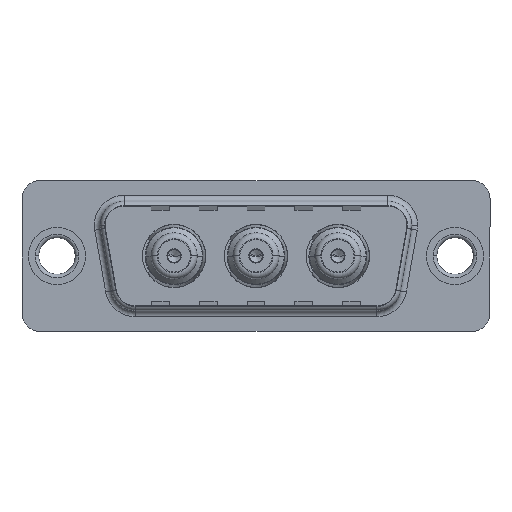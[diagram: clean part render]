
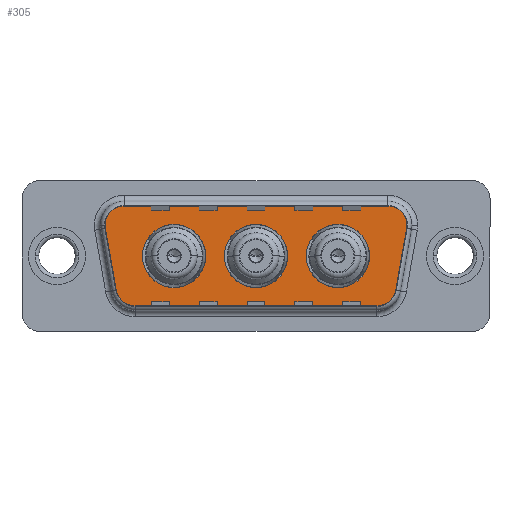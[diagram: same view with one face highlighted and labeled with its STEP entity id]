
A CAD part, top view. The second image highlights one B-rep face of the part: STEP entity #305.
In plain terms, the highlighted planar face has unit normal (0, 0, 1).
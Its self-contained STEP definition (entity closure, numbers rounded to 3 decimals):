
#219 = CIRCLE ( 'NONE', #7672, 2. ) ;
#305 = ADVANCED_FACE ( 'NONE', ( #7602, #4813, #5475, #1991 ), #2094, .T. ) ;
#312 = EDGE_CURVE ( 'NONE', #4583, #5048, #7278, .T. ) ;
#350 = EDGE_CURVE ( 'NONE', #5843, #3538, #12438, .T. ) ;
#548 = ORIENTED_EDGE ( 'NONE', *, *, #13000, .F. ) ;
#669 = VERTEX_POINT ( 'NONE', #8263 ) ;
#815 = DIRECTION ( 'NONE',  ( 1., 0., 0. ) ) ;
#873 = ORIENTED_EDGE ( 'NONE', *, *, #6352, .F. ) ;
#884 = CARTESIAN_POINT ( 'NONE',  ( 6.434, -4.9, 0. ) ) ;
#951 = CARTESIAN_POINT ( 'NONE',  ( 6.434, -4.9, 0. ) ) ;
#1049 = CARTESIAN_POINT ( 'NONE',  ( 29.889, 2.9, 0. ) ) ;
#1093 = DIRECTION ( 'NONE',  ( -1., 0., 0. ) ) ;
#1325 = DIRECTION ( 'NONE',  ( 1., 0., 0. ) ) ;
#1418 = DIRECTION ( 'NONE',  ( 0., 0., 1. ) ) ;
#1433 = CARTESIAN_POINT ( 'NONE',  ( 26.866, -2.9, 0. ) ) ;
#1539 = VERTEX_POINT ( 'NONE', #7006 ) ;
#1578 = DIRECTION ( 'NONE',  ( 0.174, -0.985, 0. ) ) ;
#1625 = CARTESIAN_POINT ( 'NONE',  ( 4.464, -3.247, 0. ) ) ;
#1694 = ORIENTED_EDGE ( 'NONE', *, *, #9275, .T. ) ;
#1715 = DIRECTION ( 'NONE',  ( 1., 0., 0. ) ) ;
#1843 = LINE ( 'NONE', #6529, #4646 ) ;
#1866 = DIRECTION ( 'NONE',  ( 0., 0., 1. ) ) ;
#1873 = ORIENTED_EDGE ( 'NONE', *, *, #350, .F. ) ;
#1991 = FACE_OUTER_BOUND ( 'NONE', #2039, .T. ) ;
#2030 = CIRCLE ( 'NONE', #5771, 2.65 ) ;
#2039 = EDGE_LOOP ( 'NONE', ( #4835, #1694, #13299, #4308, #8516, #3446, #9235, #6555, #13238 ) ) ;
#2087 = DIRECTION ( 'NONE',  ( 1., 0., 0. ) ) ;
#2094 = PLANE ( 'NONE',  #8190 ) ;
#2389 = VERTEX_POINT ( 'NONE', #4842 ) ;
#2816 = CIRCLE ( 'NONE', #4348, 2. ) ;
#3002 = EDGE_LOOP ( 'NONE', ( #873, #1873 ) ) ;
#3125 = DIRECTION ( 'NONE',  ( 0., 0., 1. ) ) ;
#3180 = VECTOR ( 'NONE', #1578, 1000. ) ;
#3446 = ORIENTED_EDGE ( 'NONE', *, *, #3728, .T. ) ;
#3448 = VERTEX_POINT ( 'NONE', #11236 ) ;
#3457 = DIRECTION ( 'NONE',  ( 0., 0., 1. ) ) ;
#3521 = LINE ( 'NONE', #4662, #3180 ) ;
#3538 = VERTEX_POINT ( 'NONE', #8340 ) ;
#3636 = VERTEX_POINT ( 'NONE', #11323 ) ;
#3728 = EDGE_CURVE ( 'NONE', #2389, #3636, #4370, .T. ) ;
#4037 = DIRECTION ( 'NONE',  ( 1., 0., 0. ) ) ;
#4214 = CARTESIAN_POINT ( 'NONE',  ( 9.8, 0., 0. ) ) ;
#4270 = CARTESIAN_POINT ( 'NONE',  ( 29.859, 2.553, 0. ) ) ;
#4308 = ORIENTED_EDGE ( 'NONE', *, *, #13515, .T. ) ;
#4348 = AXIS2_PLACEMENT_3D ( 'NONE', #1433, #1418, #1325 ) ;
#4370 = CIRCLE ( 'NONE', #12523, 2. ) ;
#4517 = VERTEX_POINT ( 'NONE', #12290 ) ;
#4583 = VERTEX_POINT ( 'NONE', #1625 ) ;
#4646 = VECTOR ( 'NONE', #6533, 1000. ) ;
#4662 = CARTESIAN_POINT ( 'NONE',  ( 3.441, 2.553, 0. ) ) ;
#4813 = FACE_BOUND ( 'NONE', #3002, .T. ) ;
#4835 = ORIENTED_EDGE ( 'NONE', *, *, #6256, .T. ) ;
#4842 = CARTESIAN_POINT ( 'NONE',  ( 5.411, 4.9, 0. ) ) ;
#5048 = VERTEX_POINT ( 'NONE', #951 ) ;
#5104 = EDGE_CURVE ( 'NONE', #3636, #4583, #3521, .T. ) ;
#5265 = EDGE_CURVE ( 'NONE', #3448, #8565, #7474, .T. ) ;
#5288 = DIRECTION ( 'NONE',  ( 1., 0., 0. ) ) ;
#5297 = DIRECTION ( 'NONE',  ( 1., 0., 0. ) ) ;
#5354 = DIRECTION ( 'NONE',  ( 0., 0., 1. ) ) ;
#5415 = CARTESIAN_POINT ( 'NONE',  ( 16.65, 0., 0. ) ) ;
#5475 = FACE_BOUND ( 'NONE', #5537, .T. ) ;
#5491 = ORIENTED_EDGE ( 'NONE', *, *, #5265, .F. ) ;
#5537 = EDGE_LOOP ( 'NONE', ( #548, #5491 ) ) ;
#5771 = AXIS2_PLACEMENT_3D ( 'NONE', #6089, #13356, #7141 ) ;
#5843 = VERTEX_POINT ( 'NONE', #10604 ) ;
#6089 = CARTESIAN_POINT ( 'NONE',  ( 16.65, 0., 0. ) ) ;
#6122 = AXIS2_PLACEMENT_3D ( 'NONE', #10112, #3457, #2087 ) ;
#6256 = EDGE_CURVE ( 'NONE', #4517, #7244, #2816, .T. ) ;
#6330 = CIRCLE ( 'NONE', #12714, 2.65 ) ;
#6352 = EDGE_CURVE ( 'NONE', #3538, #5843, #13139, .T. ) ;
#6529 = CARTESIAN_POINT ( 'NONE',  ( 5.411, 4.9, 0. ) ) ;
#6533 = DIRECTION ( 'NONE',  ( -1., 0., 0. ) ) ;
#6555 = ORIENTED_EDGE ( 'NONE', *, *, #312, .T. ) ;
#6572 = DIRECTION ( 'NONE',  ( 0., 0., 1. ) ) ;
#7006 = CARTESIAN_POINT ( 'NONE',  ( 14., 0., 0. ) ) ;
#7141 = DIRECTION ( 'NONE',  ( 1., 0., 0. ) ) ;
#7210 = LINE ( 'NONE', #884, #9903 ) ;
#7244 = VERTEX_POINT ( 'NONE', #11518 ) ;
#7278 = CIRCLE ( 'NONE', #7559, 2. ) ;
#7324 = DIRECTION ( 'NONE',  ( 0., 0., 1. ) ) ;
#7397 = EDGE_CURVE ( 'NONE', #669, #2389, #1843, .T. ) ;
#7401 = CARTESIAN_POINT ( 'NONE',  ( 19.3, 0., 0. ) ) ;
#7474 = CIRCLE ( 'NONE', #6122, 2.65 ) ;
#7559 = AXIS2_PLACEMENT_3D ( 'NONE', #8537, #8494, #1093 ) ;
#7602 = FACE_BOUND ( 'NONE', #13460, .T. ) ;
#7633 = VERTEX_POINT ( 'NONE', #1049 ) ;
#7672 = AXIS2_PLACEMENT_3D ( 'NONE', #9361, #3125, #10411 ) ;
#7714 = VECTOR ( 'NONE', #8343, 1000. ) ;
#7722 = CARTESIAN_POINT ( 'NONE',  ( 5.411, 2.9, 0. ) ) ;
#7938 = ORIENTED_EDGE ( 'NONE', *, *, #8154, .F. ) ;
#8122 = CARTESIAN_POINT ( 'NONE',  ( 27.889, 2.9, 0. ) ) ;
#8154 = EDGE_CURVE ( 'NONE', #1539, #9436, #9317, .T. ) ;
#8190 = AXIS2_PLACEMENT_3D ( 'NONE', #13122, #7324, #1715 ) ;
#8263 = CARTESIAN_POINT ( 'NONE',  ( 27.889, 4.9, 0. ) ) ;
#8340 = CARTESIAN_POINT ( 'NONE',  ( 26.15, 0., 0. ) ) ;
#8343 = DIRECTION ( 'NONE',  ( 0.174, 0.985, 0. ) ) ;
#8346 = CARTESIAN_POINT ( 'NONE',  ( 29.859, 2.553, 0. ) ) ;
#8494 = DIRECTION ( 'NONE',  ( 0., 0., 1. ) ) ;
#8516 = ORIENTED_EDGE ( 'NONE', *, *, #7397, .T. ) ;
#8537 = CARTESIAN_POINT ( 'NONE',  ( 6.434, -2.9, 0. ) ) ;
#8565 = VERTEX_POINT ( 'NONE', #12390 ) ;
#8631 = CIRCLE ( 'NONE', #10065, 2. ) ;
#9143 = DIRECTION ( 'NONE',  ( -1., 0., 0. ) ) ;
#9206 = AXIS2_PLACEMENT_3D ( 'NONE', #11810, #12424, #12400 ) ;
#9235 = ORIENTED_EDGE ( 'NONE', *, *, #5104, .T. ) ;
#9275 = EDGE_CURVE ( 'NONE', #7244, #9987, #10096, .T. ) ;
#9317 = CIRCLE ( 'NONE', #9492, 2.65 ) ;
#9361 = CARTESIAN_POINT ( 'NONE',  ( 27.889, 2.9, 0. ) ) ;
#9436 = VERTEX_POINT ( 'NONE', #7401 ) ;
#9492 = AXIS2_PLACEMENT_3D ( 'NONE', #5415, #5354, #5288 ) ;
#9585 = AXIS2_PLACEMENT_3D ( 'NONE', #13168, #9846, #9812 ) ;
#9812 = DIRECTION ( 'NONE',  ( 1., 0., 0. ) ) ;
#9846 = DIRECTION ( 'NONE',  ( 0., 0., 1. ) ) ;
#9903 = VECTOR ( 'NONE', #815, 1000. ) ;
#9987 = VERTEX_POINT ( 'NONE', #4270 ) ;
#10065 = AXIS2_PLACEMENT_3D ( 'NONE', #8122, #1866, #9143 ) ;
#10096 = LINE ( 'NONE', #8346, #7714 ) ;
#10112 = CARTESIAN_POINT ( 'NONE',  ( 9.8, 0., 0. ) ) ;
#10411 = DIRECTION ( 'NONE',  ( -1., 0., 0. ) ) ;
#10604 = CARTESIAN_POINT ( 'NONE',  ( 20.85, 0., 0. ) ) ;
#10640 = EDGE_CURVE ( 'NONE', #5048, #4517, #7210, .T. ) ;
#11236 = CARTESIAN_POINT ( 'NONE',  ( 7.15, 0., 0. ) ) ;
#11323 = CARTESIAN_POINT ( 'NONE',  ( 3.441, 2.553, 0. ) ) ;
#11477 = ORIENTED_EDGE ( 'NONE', *, *, #12852, .F. ) ;
#11484 = DIRECTION ( 'NONE',  ( 0., 0., 1. ) ) ;
#11518 = CARTESIAN_POINT ( 'NONE',  ( 28.836, -3.247, 0. ) ) ;
#11810 = CARTESIAN_POINT ( 'NONE',  ( 23.5, 0., 0. ) ) ;
#12290 = CARTESIAN_POINT ( 'NONE',  ( 26.866, -4.9, 0. ) ) ;
#12297 = EDGE_CURVE ( 'NONE', #9987, #7633, #219, .T. ) ;
#12390 = CARTESIAN_POINT ( 'NONE',  ( 12.45, 0., 0. ) ) ;
#12400 = DIRECTION ( 'NONE',  ( 1., 0., 0. ) ) ;
#12424 = DIRECTION ( 'NONE',  ( 0., 0., 1. ) ) ;
#12438 = CIRCLE ( 'NONE', #9585, 2.65 ) ;
#12523 = AXIS2_PLACEMENT_3D ( 'NONE', #7722, #6572, #4037 ) ;
#12714 = AXIS2_PLACEMENT_3D ( 'NONE', #4214, #11484, #5297 ) ;
#12852 = EDGE_CURVE ( 'NONE', #9436, #1539, #2030, .T. ) ;
#13000 = EDGE_CURVE ( 'NONE', #8565, #3448, #6330, .T. ) ;
#13122 = CARTESIAN_POINT ( 'NONE',  ( 26.866, -2.9, 0. ) ) ;
#13139 = CIRCLE ( 'NONE', #9206, 2.65 ) ;
#13168 = CARTESIAN_POINT ( 'NONE',  ( 23.5, 0., 0. ) ) ;
#13238 = ORIENTED_EDGE ( 'NONE', *, *, #10640, .T. ) ;
#13299 = ORIENTED_EDGE ( 'NONE', *, *, #12297, .T. ) ;
#13356 = DIRECTION ( 'NONE',  ( 0., 0., 1. ) ) ;
#13460 = EDGE_LOOP ( 'NONE', ( #11477, #7938 ) ) ;
#13515 = EDGE_CURVE ( 'NONE', #7633, #669, #8631, .T. ) ;
